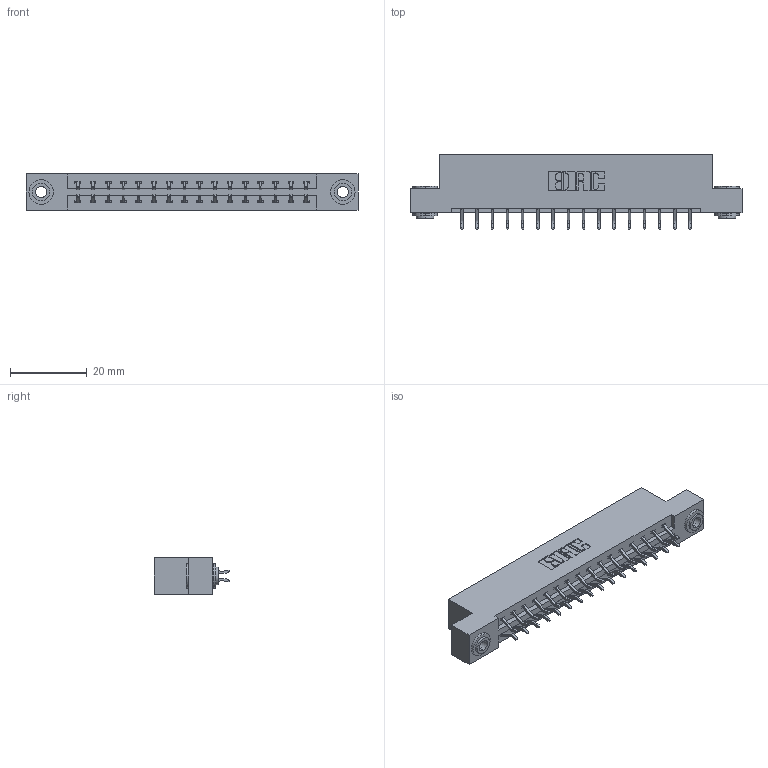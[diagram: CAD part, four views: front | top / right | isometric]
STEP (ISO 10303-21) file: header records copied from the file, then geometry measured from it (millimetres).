
FILE_DESCRIPTION (( 'STEP AP203' ), '1' );
FILE_NAME ('387-032-556-203.STEP', '2019-10-17T16:21:13', ( '' ), ( '' ), 'SwSTEP 2.0', 'SolidWorks 2016', '' );
FILE_SCHEMA (( 'CONFIG_CONTROL_DESIGN' ));
Length unit declared in the file: inch
Products named in the file (4): 345-292-001_556 Tail; 337 Part_Flush Mounting Lugs - 0.156 Dia-TH; 387-032-556-203; 345-250-002_345-250-002-102
Assembly tree (35 placements, depth 2):
  387-032-556-203
    337 Part_Flush Mounting Lugs - 0.156 Dia-TH
    345-292-001_556 Tail  x32
    345-250-002_345-250-002-102  x2
Bounding box: 86.41 x 19.57 x 9.4 mm (x, y, z)
Volume: 8778.7 mm3; surface area: 9862.4 mm2
Topology: 35 solids, 35 shells, 2072 faces, 6115 edges, 4030 vertices
Faces by surface type: plane 1424, cylinder 640, cone 8
Entity records: 16638 total; most frequent: CARTESIAN_POINT 2813, ORIENTED_EDGE 2730, DIRECTION 2463, EDGE_CURVE 1365, VECTOR 1205, LINE 1205, VERTEX_POINT 906, AXIS2_PLACEMENT_3D 629
